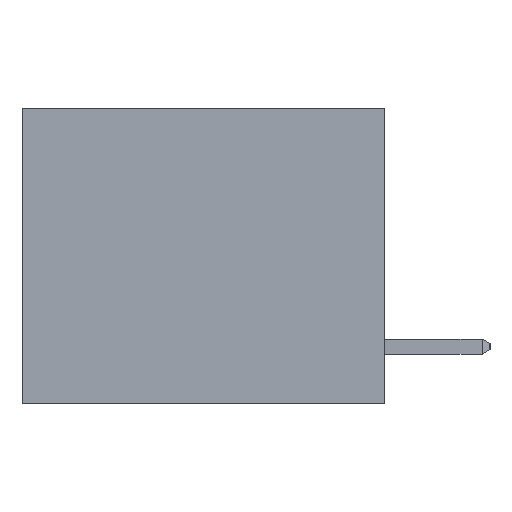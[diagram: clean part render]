
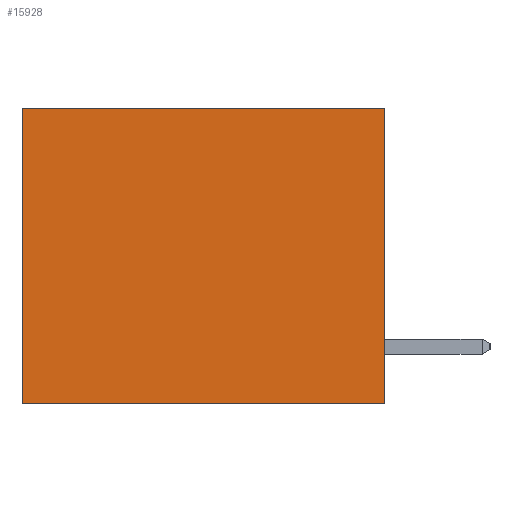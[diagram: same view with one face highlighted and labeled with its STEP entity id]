
A CAD part, left-side view. The second image highlights one B-rep face of the part: STEP entity #15928.
In plain terms, the highlighted planar face has unit normal (-1, 0, 0).
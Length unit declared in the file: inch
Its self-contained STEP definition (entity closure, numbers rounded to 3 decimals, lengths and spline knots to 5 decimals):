
#580 = VECTOR ( 'NONE', #26080, 39.37008 ) ;
#2891 = CARTESIAN_POINT ( 'NONE',  ( 0.3165, 0., 0. ) ) ;
#3238 = ORIENTED_EDGE ( 'NONE', *, *, #23598, .T. ) ;
#3925 = LINE ( 'NONE', #19643, #580 ) ;
#4208 = LINE ( 'NONE', #19427, #12087 ) ;
#5783 = CARTESIAN_POINT ( 'NONE',  ( 0.3165, 0., -0.49 ) ) ;
#7718 = AXIS2_PLACEMENT_3D ( 'NONE', #13596, #19900, #19528 ) ;
#8781 = VERTEX_POINT ( 'NONE', #25173 ) ;
#11178 = LINE ( 'NONE', #20407, #22427 ) ;
#12087 = VECTOR ( 'NONE', #14905, 39.37008 ) ;
#13183 = VERTEX_POINT ( 'NONE', #16841 ) ;
#13408 = FACE_OUTER_BOUND ( 'NONE', #19588, .T. ) ;
#13596 = CARTESIAN_POINT ( 'NONE',  ( 0.3165, 0., -0.49 ) ) ;
#13959 = CARTESIAN_POINT ( 'NONE',  ( 0.3165, 0., -0.49 ) ) ;
#14808 = LINE ( 'NONE', #5783, #21424 ) ;
#14905 = DIRECTION ( 'NONE',  ( 0., 0., -1. ) ) ;
#15651 = PLANE ( 'NONE',  #7718 ) ;
#15788 = EDGE_CURVE ( 'NONE', #19188, #26528, #4208, .T. ) ;
#15928 = ADVANCED_FACE ( 'NONE', ( #13408 ), #15651, .F. ) ;
#16371 = ORIENTED_EDGE ( 'NONE', *, *, #20140, .F. ) ;
#16841 = CARTESIAN_POINT ( 'NONE',  ( 0.3165, 0.6, 0. ) ) ;
#17108 = ORIENTED_EDGE ( 'NONE', *, *, #15788, .F. ) ;
#18166 = ORIENTED_EDGE ( 'NONE', *, *, #20633, .T. ) ;
#18171 = DIRECTION ( 'NONE',  ( 0., 0., -1. ) ) ;
#19188 = VERTEX_POINT ( 'NONE', #2891 ) ;
#19427 = CARTESIAN_POINT ( 'NONE',  ( 0.3165, 0., -0.49 ) ) ;
#19528 = DIRECTION ( 'NONE',  ( 0., 0., -1. ) ) ;
#19588 = EDGE_LOOP ( 'NONE', ( #18166, #16371, #17108, #3238 ) ) ;
#19643 = CARTESIAN_POINT ( 'NONE',  ( 0.3165, 0., 0. ) ) ;
#19900 = DIRECTION ( 'NONE',  ( 1., 0., 0. ) ) ;
#20140 = EDGE_CURVE ( 'NONE', #26528, #8781, #14808, .T. ) ;
#20407 = CARTESIAN_POINT ( 'NONE',  ( 0.3165, 0.6, -0.49 ) ) ;
#20633 = EDGE_CURVE ( 'NONE', #13183, #8781, #11178, .T. ) ;
#21424 = VECTOR ( 'NONE', #22460, 39.37008 ) ;
#22427 = VECTOR ( 'NONE', #18171, 39.37008 ) ;
#22460 = DIRECTION ( 'NONE',  ( 0., 1., 0. ) ) ;
#23598 = EDGE_CURVE ( 'NONE', #19188, #13183, #3925, .T. ) ;
#25173 = CARTESIAN_POINT ( 'NONE',  ( 0.3165, 0.6, -0.49 ) ) ;
#26080 = DIRECTION ( 'NONE',  ( 0., 1., 0. ) ) ;
#26528 = VERTEX_POINT ( 'NONE', #13959 ) ;
